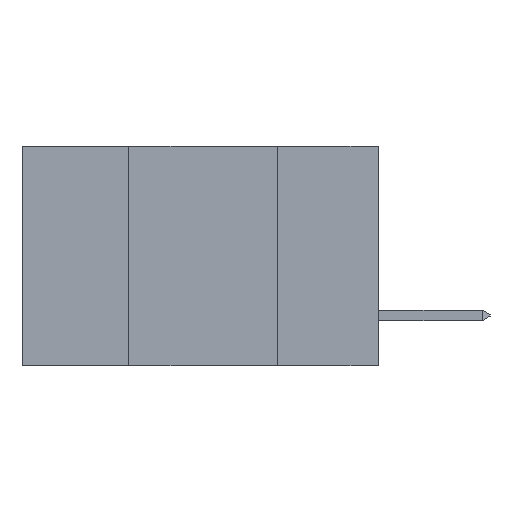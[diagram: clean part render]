
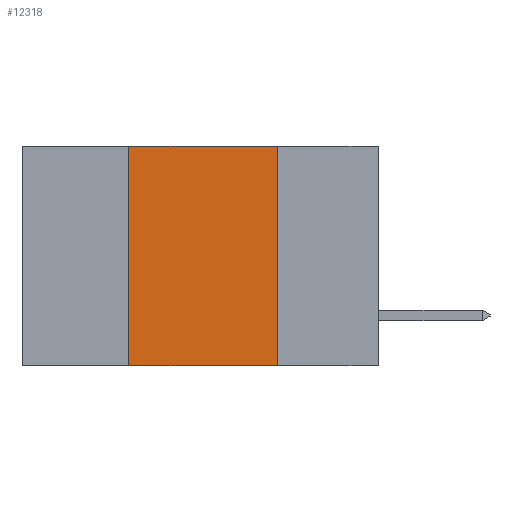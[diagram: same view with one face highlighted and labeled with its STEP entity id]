
A CAD part, left-side view. The second image highlights one B-rep face of the part: STEP entity #12318.
In plain terms, the highlighted planar face has unit normal (-1, 0, 0).
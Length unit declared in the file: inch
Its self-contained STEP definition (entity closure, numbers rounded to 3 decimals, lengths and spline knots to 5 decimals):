
#668 = VECTOR ( 'NONE', #6720, 39.37008 ) ;
#871 = ORIENTED_EDGE ( 'NONE', *, *, #12316, .T. ) ;
#959 = CARTESIAN_POINT ( 'NONE',  ( 0., 0.6, 0. ) ) ;
#1458 = VERTEX_POINT ( 'NONE', #12682 ) ;
#1727 = ORIENTED_EDGE ( 'NONE', *, *, #12934, .F. ) ;
#2051 = DIRECTION ( 'NONE',  ( 1., 0., 0. ) ) ;
#2071 = ORIENTED_EDGE ( 'NONE', *, *, #5452, .F. ) ;
#2201 = FACE_OUTER_BOUND ( 'NONE', #3502, .T. ) ;
#2456 = EDGE_CURVE ( 'NONE', #1458, #7341, #8495, .T. ) ;
#2589 = CARTESIAN_POINT ( 'NONE',  ( 0., 0.42, -0.37 ) ) ;
#3041 = ORIENTED_EDGE ( 'NONE', *, *, #2456, .F. ) ;
#3317 = LINE ( 'NONE', #11893, #8390 ) ;
#3420 = CARTESIAN_POINT ( 'NONE',  ( 0., 0.17, -0.37 ) ) ;
#3502 = EDGE_LOOP ( 'NONE', ( #3041, #2071, #1727, #871 ) ) ;
#3535 = LINE ( 'NONE', #11603, #668 ) ;
#4382 = CARTESIAN_POINT ( 'NONE',  ( 0., 0.17, -0.37 ) ) ;
#4392 = DIRECTION ( 'NONE',  ( 0., 0., -1. ) ) ;
#4423 = VECTOR ( 'NONE', #4392, 39.37008 ) ;
#5020 = DIRECTION ( 'NONE',  ( 0., 0., 1. ) ) ;
#5452 = EDGE_CURVE ( 'NONE', #10380, #1458, #3535, .T. ) ;
#6298 = VERTEX_POINT ( 'NONE', #2589 ) ;
#6720 = DIRECTION ( 'NONE',  ( 0., -1., 0. ) ) ;
#7134 = DIRECTION ( 'NONE',  ( 0., -1., 0. ) ) ;
#7341 = VERTEX_POINT ( 'NONE', #3420 ) ;
#7624 = LINE ( 'NONE', #12026, #12510 ) ;
#8166 = PLANE ( 'NONE',  #8653 ) ;
#8390 = VECTOR ( 'NONE', #5020, 39.37008 ) ;
#8495 = LINE ( 'NONE', #4382, #4423 ) ;
#8636 = CARTESIAN_POINT ( 'NONE',  ( 0., 0.42, 0. ) ) ;
#8653 = AXIS2_PLACEMENT_3D ( 'NONE', #959, #2051, #9149 ) ;
#9149 = DIRECTION ( 'NONE',  ( 0., 0., -1. ) ) ;
#10380 = VERTEX_POINT ( 'NONE', #8636 ) ;
#11603 = CARTESIAN_POINT ( 'NONE',  ( 0., 0.6, 0. ) ) ;
#11893 = CARTESIAN_POINT ( 'NONE',  ( 0., 0.42, -0.37 ) ) ;
#12026 = CARTESIAN_POINT ( 'NONE',  ( 0., 0.6, -0.37 ) ) ;
#12316 = EDGE_CURVE ( 'NONE', #6298, #7341, #7624, .T. ) ;
#12318 = ADVANCED_FACE ( 'NONE', ( #2201 ), #8166, .F. ) ;
#12510 = VECTOR ( 'NONE', #7134, 39.37008 ) ;
#12682 = CARTESIAN_POINT ( 'NONE',  ( 0., 0.17, 0. ) ) ;
#12934 = EDGE_CURVE ( 'NONE', #6298, #10380, #3317, .T. ) ;
